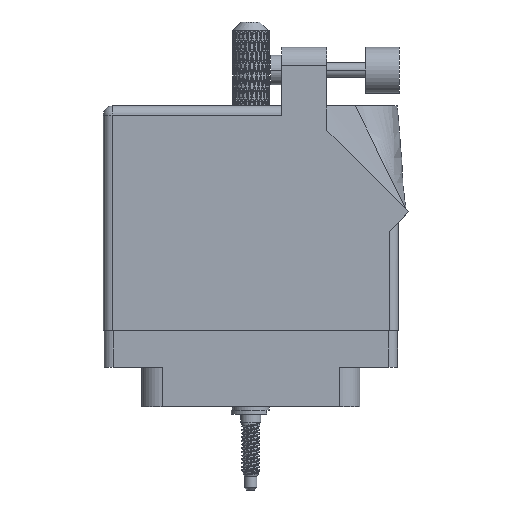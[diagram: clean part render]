
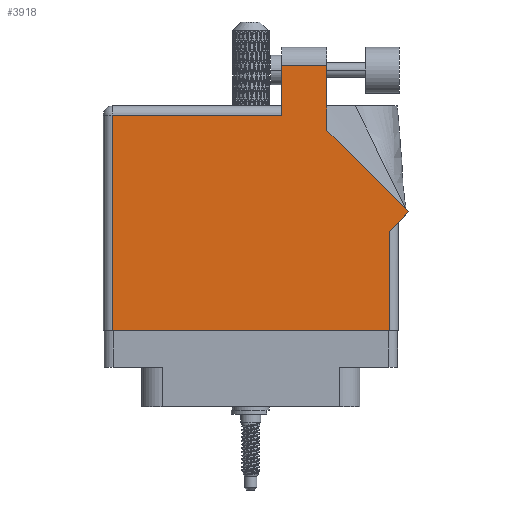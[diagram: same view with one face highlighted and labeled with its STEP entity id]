
A CAD part, front view. The second image highlights one B-rep face of the part: STEP entity #3918.
In plain terms, the highlighted face is planar.
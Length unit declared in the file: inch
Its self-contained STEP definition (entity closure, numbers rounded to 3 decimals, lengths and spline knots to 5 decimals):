
#126 = CARTESIAN_POINT ( 'NONE',  ( 1.005, 0.637, 0.455 ) ) ;
#1354 = VECTOR ( 'NONE', #59018, 39.37008 ) ;
#3575 = CARTESIAN_POINT ( 'NONE',  ( -1.005, 1.43, 0.455 ) ) ;
#3734 = CARTESIAN_POINT ( 'NONE',  ( 1.07571, 0.70771, 0.455 ) ) ;
#3918 = ADVANCED_FACE ( 'NONE', ( #21832 ), #27935, .F. ) ;
#4703 = LINE ( 'NONE', #26186, #85938 ) ;
#5710 = VECTOR ( 'NONE', #89833, 39.37008 ) ;
#7423 = CARTESIAN_POINT ( 'NONE',  ( 0.943, 0.637, 0.455 ) ) ;
#17984 = ORIENTED_EDGE ( 'NONE', *, *, #29873, .T. ) ;
#18820 = CARTESIAN_POINT ( 'NONE',  ( -1.005, 1.368, 0.455 ) ) ;
#21832 = FACE_OUTER_BOUND ( 'NONE', #91674, .T. ) ;
#26186 = CARTESIAN_POINT ( 'NONE',  ( 0.212, 1.43, 0.455 ) ) ;
#26506 = CARTESIAN_POINT ( 'NONE',  ( -0.943, -0.1, 0.455 ) ) ;
#26919 = LINE ( 'NONE', #7423, #83525 ) ;
#27173 = DIRECTION ( 'NONE',  ( 0., -1., 0. ) ) ;
#27752 = EDGE_CURVE ( 'NONE', #101761, #42588, #26919, .T. ) ;
#27935 = PLANE ( 'NONE',  #32336 ) ;
#29842 = CARTESIAN_POINT ( 'NONE',  ( 0.519, 1.26442, 0.455 ) ) ;
#29873 = EDGE_CURVE ( 'NONE', #74367, #47641, #71525, .T. ) ;
#30359 = ORIENTED_EDGE ( 'NONE', *, *, #47828, .T. ) ;
#31101 = ORIENTED_EDGE ( 'NONE', *, *, #91313, .T. ) ;
#31176 = VECTOR ( 'NONE', #91182, 39.37008 ) ;
#31337 = CARTESIAN_POINT ( 'NONE',  ( -0.943, -0.1, 0.455 ) ) ;
#32336 = AXIS2_PLACEMENT_3D ( 'NONE', #3575, #74754, #91279 ) ;
#35331 = DIRECTION ( 'NONE',  ( -0.707, 0.707, 0. ) ) ;
#36473 = LINE ( 'NONE', #26506, #5710 ) ;
#38349 = VERTEX_POINT ( 'NONE', #29842 ) ;
#39965 = DIRECTION ( 'NONE',  ( 0.707, 0.707, 0. ) ) ;
#40608 = ORIENTED_EDGE ( 'NONE', *, *, #56856, .T. ) ;
#42588 = VERTEX_POINT ( 'NONE', #89482 ) ;
#45486 = VERTEX_POINT ( 'NONE', #91555 ) ;
#45801 = LINE ( 'NONE', #3734, #88971 ) ;
#46612 = EDGE_CURVE ( 'NONE', #91214, #101761, #68141, .T. ) ;
#47641 = VERTEX_POINT ( 'NONE', #85671 ) ;
#47828 = EDGE_CURVE ( 'NONE', #45486, #38349, #45801, .T. ) ;
#49318 = VECTOR ( 'NONE', #39965, 39.37008 ) ;
#49546 = VERTEX_POINT ( 'NONE', #61108 ) ;
#50239 = EDGE_CURVE ( 'NONE', #47641, #49546, #4703, .T. ) ;
#51443 = CARTESIAN_POINT ( 'NONE',  ( 0.519, 1.26442, 0.455 ) ) ;
#51929 = ORIENTED_EDGE ( 'NONE', *, *, #75346, .T. ) ;
#55272 = CARTESIAN_POINT ( 'NONE',  ( -0.943, 1.368, 0.455 ) ) ;
#56856 = EDGE_CURVE ( 'NONE', #38349, #74367, #101050, .T. ) ;
#57179 = ORIENTED_EDGE ( 'NONE', *, *, #70401, .T. ) ;
#58281 = CARTESIAN_POINT ( 'NONE',  ( 0.212, 1.705, 0.455 ) ) ;
#58437 = CARTESIAN_POINT ( 'NONE',  ( 0.943, -0.1, 0.455 ) ) ;
#59018 = DIRECTION ( 'NONE',  ( 0., 1., 0. ) ) ;
#59487 = CARTESIAN_POINT ( 'NONE',  ( -1.005, -0.1, 0.455 ) ) ;
#61108 = CARTESIAN_POINT ( 'NONE',  ( 0.212, 1.368, 0.455 ) ) ;
#62738 = DIRECTION ( 'NONE',  ( 0., 1., 0. ) ) ;
#63442 = VERTEX_POINT ( 'NONE', #55272 ) ;
#67002 = ORIENTED_EDGE ( 'NONE', *, *, #27752, .T. ) ;
#68141 = LINE ( 'NONE', #59487, #31176 ) ;
#69722 = CARTESIAN_POINT ( 'NONE',  ( 0.519, 1.705, 0.455 ) ) ;
#70240 = LINE ( 'NONE', #126, #49318 ) ;
#70318 = VECTOR ( 'NONE', #83830, 39.37008 ) ;
#70401 = EDGE_CURVE ( 'NONE', #49546, #63442, #74009, .T. ) ;
#70463 = ORIENTED_EDGE ( 'NONE', *, *, #50239, .T. ) ;
#71525 = LINE ( 'NONE', #58281, #76382 ) ;
#74009 = LINE ( 'NONE', #18820, #70318 ) ;
#74367 = VERTEX_POINT ( 'NONE', #69722 ) ;
#74754 = DIRECTION ( 'NONE',  ( 0., 0., -1. ) ) ;
#74935 = ORIENTED_EDGE ( 'NONE', *, *, #46612, .T. ) ;
#75346 = EDGE_CURVE ( 'NONE', #42588, #45486, #70240, .T. ) ;
#76382 = VECTOR ( 'NONE', #82399, 39.37008 ) ;
#82399 = DIRECTION ( 'NONE',  ( -1., 0., 0. ) ) ;
#83525 = VECTOR ( 'NONE', #62738, 39.37008 ) ;
#83830 = DIRECTION ( 'NONE',  ( -1., 0., 0. ) ) ;
#85671 = CARTESIAN_POINT ( 'NONE',  ( 0.212, 1.705, 0.455 ) ) ;
#85938 = VECTOR ( 'NONE', #27173, 39.37008 ) ;
#88971 = VECTOR ( 'NONE', #35331, 39.37008 ) ;
#89482 = CARTESIAN_POINT ( 'NONE',  ( 0.943, 0.575, 0.455 ) ) ;
#89833 = DIRECTION ( 'NONE',  ( 0., -1., 0. ) ) ;
#91182 = DIRECTION ( 'NONE',  ( 1., 0., 0. ) ) ;
#91214 = VERTEX_POINT ( 'NONE', #31337 ) ;
#91279 = DIRECTION ( 'NONE',  ( -1., 0., 0. ) ) ;
#91313 = EDGE_CURVE ( 'NONE', #63442, #91214, #36473, .T. ) ;
#91555 = CARTESIAN_POINT ( 'NONE',  ( 1.07571, 0.70771, 0.455 ) ) ;
#91674 = EDGE_LOOP ( 'NONE', ( #40608, #17984, #70463, #57179, #31101, #74935, #67002, #51929, #30359 ) ) ;
#101050 = LINE ( 'NONE', #51443, #1354 ) ;
#101761 = VERTEX_POINT ( 'NONE', #58437 ) ;
